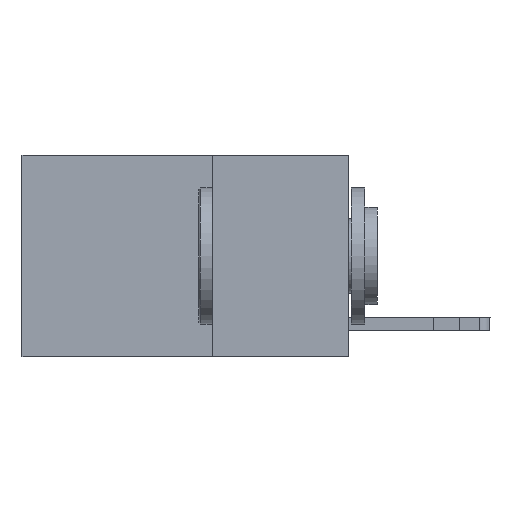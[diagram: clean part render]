
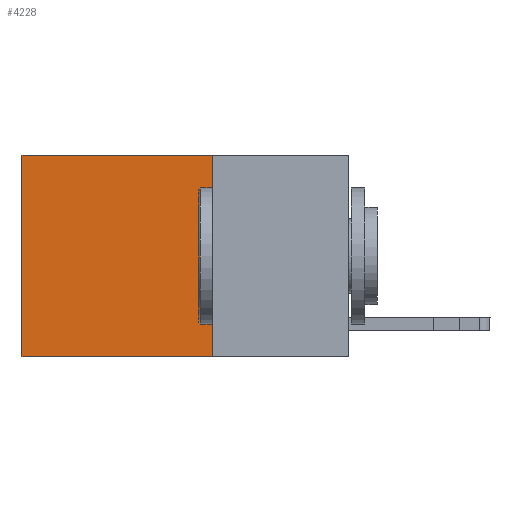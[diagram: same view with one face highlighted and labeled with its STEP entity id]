
A CAD part, left-side view. The second image highlights one B-rep face of the part: STEP entity #4228.
In plain terms, the highlighted planar face has unit normal (-1, 0, 0).
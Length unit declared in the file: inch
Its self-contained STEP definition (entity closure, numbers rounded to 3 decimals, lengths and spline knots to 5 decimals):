
#295 = VECTOR ( 'NONE', #17850, 39.37008 ) ;
#928 = CARTESIAN_POINT ( 'NONE',  ( 0.2625, 0.25, 0. ) ) ;
#1296 = DIRECTION ( 'NONE',  ( 1., 0., 0. ) ) ;
#1768 = DIRECTION ( 'NONE',  ( 0., 0., -1. ) ) ;
#2006 = VECTOR ( 'NONE', #6780, 39.37008 ) ;
#2387 = EDGE_LOOP ( 'NONE', ( #7180, #11614, #4255, #10277 ) ) ;
#2460 = VERTEX_POINT ( 'NONE', #3901 ) ;
#3901 = CARTESIAN_POINT ( 'NONE',  ( 0.2625, 0.6, 0. ) ) ;
#4032 = VECTOR ( 'NONE', #16273, 39.37008 ) ;
#4228 = ADVANCED_FACE ( 'NONE', ( #15889 ), #6875, .F. ) ;
#4255 = ORIENTED_EDGE ( 'NONE', *, *, #5367, .F. ) ;
#4361 = DIRECTION ( 'NONE',  ( 0., 0., -1. ) ) ;
#4474 = EDGE_CURVE ( 'NONE', #15024, #8794, #17712, .T. ) ;
#4563 = LINE ( 'NONE', #14841, #8519 ) ;
#5367 = EDGE_CURVE ( 'NONE', #16573, #15024, #13985, .T. ) ;
#5522 = CARTESIAN_POINT ( 'NONE',  ( 0.2625, 0.25, 0. ) ) ;
#6780 = DIRECTION ( 'NONE',  ( 0., 0., -1. ) ) ;
#6875 = PLANE ( 'NONE',  #11665 ) ;
#7180 = ORIENTED_EDGE ( 'NONE', *, *, #17621, .T. ) ;
#8519 = VECTOR ( 'NONE', #1768, 39.37008 ) ;
#8794 = VERTEX_POINT ( 'NONE', #14067 ) ;
#9048 = EDGE_CURVE ( 'NONE', #16573, #2460, #15156, .T. ) ;
#10277 = ORIENTED_EDGE ( 'NONE', *, *, #9048, .T. ) ;
#10646 = CARTESIAN_POINT ( 'NONE',  ( 0.2625, 0.25, -0.37 ) ) ;
#11614 = ORIENTED_EDGE ( 'NONE', *, *, #4474, .F. ) ;
#11665 = AXIS2_PLACEMENT_3D ( 'NONE', #5522, #1296, #4361 ) ;
#13305 = CARTESIAN_POINT ( 'NONE',  ( 0.2625, 0.25, 0. ) ) ;
#13985 = LINE ( 'NONE', #928, #2006 ) ;
#14067 = CARTESIAN_POINT ( 'NONE',  ( 0.2625, 0.6, -0.37 ) ) ;
#14841 = CARTESIAN_POINT ( 'NONE',  ( 0.2625, 0.6, 0. ) ) ;
#15024 = VERTEX_POINT ( 'NONE', #16851 ) ;
#15156 = LINE ( 'NONE', #18130, #295 ) ;
#15889 = FACE_OUTER_BOUND ( 'NONE', #2387, .T. ) ;
#16273 = DIRECTION ( 'NONE',  ( 0., 1., 0. ) ) ;
#16573 = VERTEX_POINT ( 'NONE', #13305 ) ;
#16851 = CARTESIAN_POINT ( 'NONE',  ( 0.2625, 0.25, -0.37 ) ) ;
#17621 = EDGE_CURVE ( 'NONE', #2460, #8794, #4563, .T. ) ;
#17712 = LINE ( 'NONE', #10646, #4032 ) ;
#17850 = DIRECTION ( 'NONE',  ( 0., 1., 0. ) ) ;
#18130 = CARTESIAN_POINT ( 'NONE',  ( 0.2625, 0.25, 0. ) ) ;
